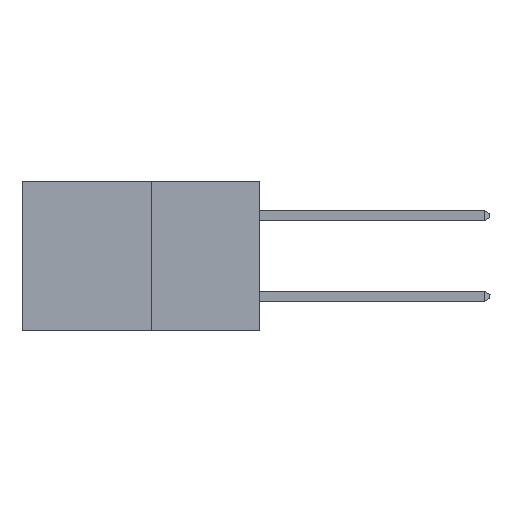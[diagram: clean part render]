
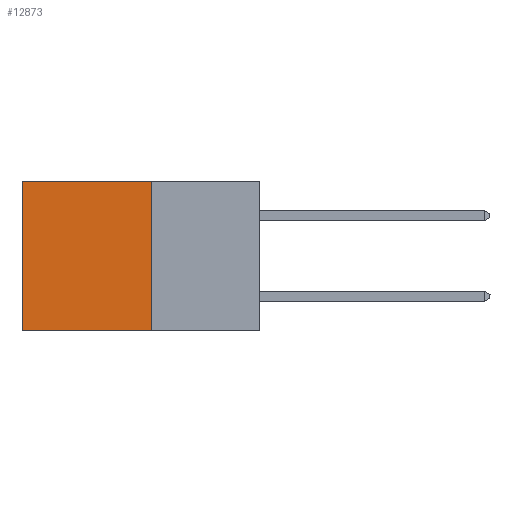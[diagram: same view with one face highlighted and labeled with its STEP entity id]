
A CAD part, left-side view. The second image highlights one B-rep face of the part: STEP entity #12873.
In plain terms, the highlighted planar face has unit normal (-1, 0, 0).
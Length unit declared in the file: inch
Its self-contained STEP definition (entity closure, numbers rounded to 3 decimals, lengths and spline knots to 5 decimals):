
#44 = CARTESIAN_POINT ( 'NONE',  ( 0.277, 0.27, -0.37 ) ) ;
#194 = PLANE ( 'NONE',  #3161 ) ;
#273 = DIRECTION ( 'NONE',  ( 0., 1., 0. ) ) ;
#691 = CARTESIAN_POINT ( 'NONE',  ( 0.277, 0.59, 0. ) ) ;
#1245 = VECTOR ( 'NONE', #9708, 39.37008 ) ;
#1874 = CARTESIAN_POINT ( 'NONE',  ( 0.277, 0.27, -0.37 ) ) ;
#1943 = DIRECTION ( 'NONE',  ( 0., 0., -1. ) ) ;
#2848 = VERTEX_POINT ( 'NONE', #11948 ) ;
#2876 = VECTOR ( 'NONE', #9028, 39.37008 ) ;
#3161 = AXIS2_PLACEMENT_3D ( 'NONE', #1874, #11755, #1943 ) ;
#3727 = VERTEX_POINT ( 'NONE', #19282 ) ;
#4920 = VECTOR ( 'NONE', #273, 39.37008 ) ;
#5908 = DIRECTION ( 'NONE',  ( 0., 1., 0. ) ) ;
#6822 = EDGE_CURVE ( 'NONE', #3727, #12828, #7267, .T. ) ;
#7267 = LINE ( 'NONE', #9076, #2876 ) ;
#7665 = EDGE_CURVE ( 'NONE', #12828, #2848, #9800, .T. ) ;
#8694 = ORIENTED_EDGE ( 'NONE', *, *, #7665, .F. ) ;
#9028 = DIRECTION ( 'NONE',  ( 0., 0., -1. ) ) ;
#9076 = CARTESIAN_POINT ( 'NONE',  ( 0.277, 0.27, -0.37 ) ) ;
#9307 = FACE_OUTER_BOUND ( 'NONE', #20629, .T. ) ;
#9708 = DIRECTION ( 'NONE',  ( 0., 0., -1. ) ) ;
#9800 = LINE ( 'NONE', #44, #4920 ) ;
#11755 = DIRECTION ( 'NONE',  ( 1., 0., 0. ) ) ;
#11948 = CARTESIAN_POINT ( 'NONE',  ( 0.277, 0.59, -0.37 ) ) ;
#12413 = VECTOR ( 'NONE', #5908, 39.37008 ) ;
#12828 = VERTEX_POINT ( 'NONE', #16331 ) ;
#12873 = ADVANCED_FACE ( 'NONE', ( #9307 ), #194, .F. ) ;
#12914 = LINE ( 'NONE', #17061, #12413 ) ;
#13714 = ORIENTED_EDGE ( 'NONE', *, *, #17072, .T. ) ;
#13816 = VERTEX_POINT ( 'NONE', #691 ) ;
#16331 = CARTESIAN_POINT ( 'NONE',  ( 0.277, 0.27, -0.37 ) ) ;
#16852 = ORIENTED_EDGE ( 'NONE', *, *, #19174, .T. ) ;
#17061 = CARTESIAN_POINT ( 'NONE',  ( 0.277, 0.27, 0. ) ) ;
#17072 = EDGE_CURVE ( 'NONE', #3727, #13816, #12914, .T. ) ;
#17378 = LINE ( 'NONE', #17530, #1245 ) ;
#17530 = CARTESIAN_POINT ( 'NONE',  ( 0.277, 0.59, -0.37 ) ) ;
#18696 = ORIENTED_EDGE ( 'NONE', *, *, #6822, .F. ) ;
#19174 = EDGE_CURVE ( 'NONE', #13816, #2848, #17378, .T. ) ;
#19282 = CARTESIAN_POINT ( 'NONE',  ( 0.277, 0.27, 0. ) ) ;
#20629 = EDGE_LOOP ( 'NONE', ( #16852, #8694, #18696, #13714 ) ) ;
